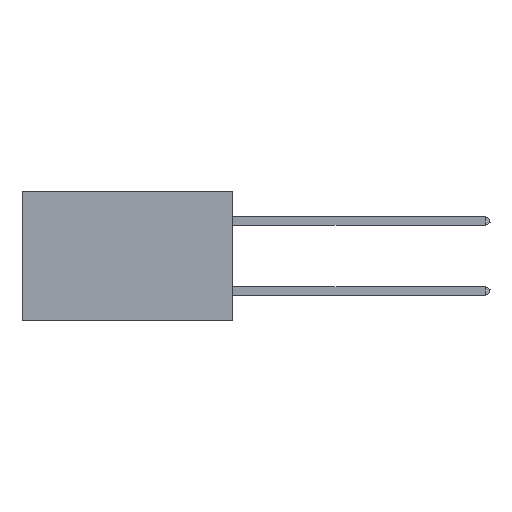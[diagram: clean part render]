
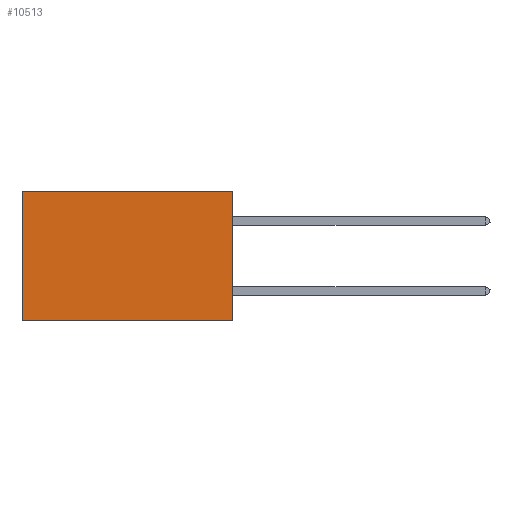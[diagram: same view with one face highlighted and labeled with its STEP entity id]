
A CAD part, left-side view. The second image highlights one B-rep face of the part: STEP entity #10513.
In plain terms, the highlighted planar face has unit normal (-1, 0, 0).
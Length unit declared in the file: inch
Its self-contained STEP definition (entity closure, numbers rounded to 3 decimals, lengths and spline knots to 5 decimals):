
#938 = DIRECTION ( 'NONE',  ( 0., 1., 0. ) ) ;
#1126 = CARTESIAN_POINT ( 'NONE',  ( 0.2875, 0., -0.37 ) ) ;
#1437 = AXIS2_PLACEMENT_3D ( 'NONE', #12908, #3368, #14398 ) ;
#1732 = PLANE ( 'NONE',  #1437 ) ;
#2010 = VERTEX_POINT ( 'NONE', #8884 ) ;
#2129 = EDGE_CURVE ( 'NONE', #2010, #10249, #2830, .T. ) ;
#2707 = FACE_OUTER_BOUND ( 'NONE', #20034, .T. ) ;
#2830 = LINE ( 'NONE', #1126, #3334 ) ;
#3334 = VECTOR ( 'NONE', #12379, 39.37008 ) ;
#3368 = DIRECTION ( 'NONE',  ( 1., 0., 0. ) ) ;
#5212 = ORIENTED_EDGE ( 'NONE', *, *, #14951, .T. ) ;
#5415 = CARTESIAN_POINT ( 'NONE',  ( 0.2875, 0., 0. ) ) ;
#5829 = CARTESIAN_POINT ( 'NONE',  ( 0.2875, 0., 0. ) ) ;
#5917 = CARTESIAN_POINT ( 'NONE',  ( 0.2875, 0.6, -0.37 ) ) ;
#6685 = EDGE_CURVE ( 'NONE', #17233, #2010, #14446, .T. ) ;
#7590 = VECTOR ( 'NONE', #938, 39.37008 ) ;
#8884 = CARTESIAN_POINT ( 'NONE',  ( 0.2875, 0., -0.37 ) ) ;
#9285 = CARTESIAN_POINT ( 'NONE',  ( 0.2875, 0.6, 0. ) ) ;
#9757 = ORIENTED_EDGE ( 'NONE', *, *, #6685, .F. ) ;
#10249 = VERTEX_POINT ( 'NONE', #5917 ) ;
#10513 = ADVANCED_FACE ( 'NONE', ( #2707 ), #1732, .F. ) ;
#11458 = CARTESIAN_POINT ( 'NONE',  ( 0.2875, 0.6, 0. ) ) ;
#11572 = DIRECTION ( 'NONE',  ( 0., 0., -1. ) ) ;
#12375 = VERTEX_POINT ( 'NONE', #9285 ) ;
#12379 = DIRECTION ( 'NONE',  ( 0., 1., 0. ) ) ;
#12908 = CARTESIAN_POINT ( 'NONE',  ( 0.2875, 0., 0. ) ) ;
#12998 = DIRECTION ( 'NONE',  ( 0., 0., -1. ) ) ;
#14097 = ORIENTED_EDGE ( 'NONE', *, *, #2129, .F. ) ;
#14398 = DIRECTION ( 'NONE',  ( 0., 0., -1. ) ) ;
#14446 = LINE ( 'NONE', #5415, #17928 ) ;
#14951 = EDGE_CURVE ( 'NONE', #17233, #12375, #19274, .T. ) ;
#15138 = VECTOR ( 'NONE', #12998, 39.37008 ) ;
#15571 = ORIENTED_EDGE ( 'NONE', *, *, #18885, .T. ) ;
#17233 = VERTEX_POINT ( 'NONE', #18121 ) ;
#17928 = VECTOR ( 'NONE', #11572, 39.37008 ) ;
#18121 = CARTESIAN_POINT ( 'NONE',  ( 0.2875, 0., 0. ) ) ;
#18885 = EDGE_CURVE ( 'NONE', #12375, #10249, #19070, .T. ) ;
#19070 = LINE ( 'NONE', #11458, #15138 ) ;
#19274 = LINE ( 'NONE', #5829, #7590 ) ;
#20034 = EDGE_LOOP ( 'NONE', ( #15571, #14097, #9757, #5212 ) ) ;
